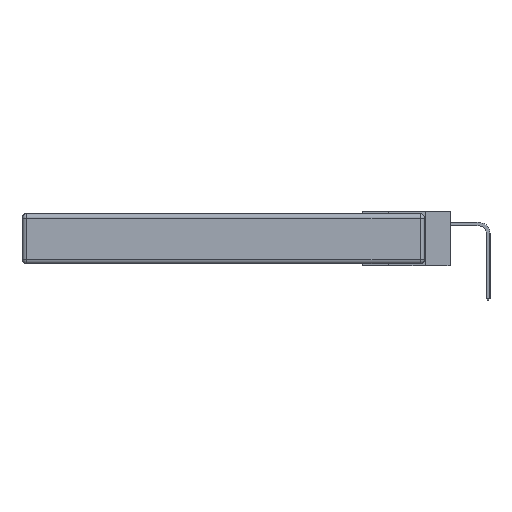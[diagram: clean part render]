
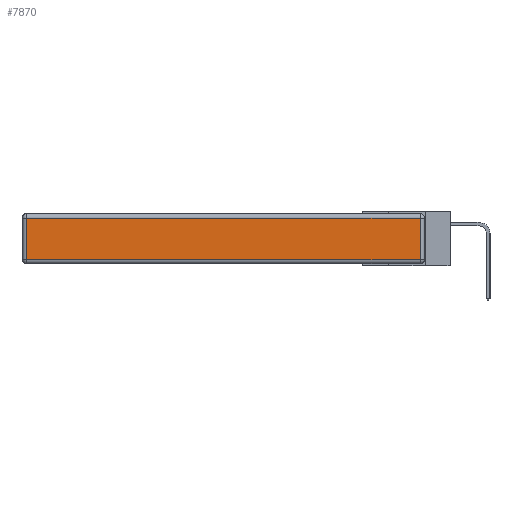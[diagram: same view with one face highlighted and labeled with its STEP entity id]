
A CAD part, left-side view. The second image highlights one B-rep face of the part: STEP entity #7870.
In plain terms, the highlighted planar face has unit normal (-1, 0, 0).
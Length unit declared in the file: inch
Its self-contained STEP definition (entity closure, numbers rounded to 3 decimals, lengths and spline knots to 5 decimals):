
#956 = VECTOR ( 'NONE', #12229, 39.37008 ) ;
#3264 = AXIS2_PLACEMENT_3D ( 'NONE', #3425, #10916, #8335 ) ;
#3312 = PLANE ( 'NONE',  #3264 ) ;
#3425 = CARTESIAN_POINT ( 'NONE',  ( 0., 0., -0.343 ) ) ;
#4411 = CARTESIAN_POINT ( 'NONE',  ( 0., 2.72, -0.03 ) ) ;
#5240 = DIRECTION ( 'NONE',  ( 0., 0., -1. ) ) ;
#5314 = LINE ( 'NONE', #24860, #31729 ) ;
#6458 = ORIENTED_EDGE ( 'NONE', *, *, #26050, .T. ) ;
#7370 = CARTESIAN_POINT ( 'NONE',  ( 0., 2.75, -0.03 ) ) ;
#7870 = ADVANCED_FACE ( 'NONE', ( #29804 ), #3312, .T. ) ;
#8335 = DIRECTION ( 'NONE',  ( 0., 0., 1. ) ) ;
#8623 = LINE ( 'NONE', #7370, #16693 ) ;
#8776 = VERTEX_POINT ( 'NONE', #24275 ) ;
#10916 = DIRECTION ( 'NONE',  ( -1., 0., 0. ) ) ;
#11237 = LINE ( 'NONE', #15755, #22353 ) ;
#12127 = CARTESIAN_POINT ( 'NONE',  ( 0., 0., -0.313 ) ) ;
#12229 = DIRECTION ( 'NONE',  ( 0., -1., 0. ) ) ;
#12957 = VERTEX_POINT ( 'NONE', #16671 ) ;
#13455 = VERTEX_POINT ( 'NONE', #13497 ) ;
#13497 = CARTESIAN_POINT ( 'NONE',  ( 0., 0.03, -0.313 ) ) ;
#15755 = CARTESIAN_POINT ( 'NONE',  ( 0., 0.03, -0.343 ) ) ;
#16356 = VERTEX_POINT ( 'NONE', #4411 ) ;
#16671 = CARTESIAN_POINT ( 'NONE',  ( 0., 0.03, -0.03 ) ) ;
#16693 = VECTOR ( 'NONE', #22162, 39.37008 ) ;
#20023 = ORIENTED_EDGE ( 'NONE', *, *, #26018, .T. ) ;
#20680 = DIRECTION ( 'NONE',  ( 0., 0., 1. ) ) ;
#21507 = ORIENTED_EDGE ( 'NONE', *, *, #23177, .T. ) ;
#22162 = DIRECTION ( 'NONE',  ( 0., 1., 0. ) ) ;
#22353 = VECTOR ( 'NONE', #20680, 39.37008 ) ;
#23177 = EDGE_CURVE ( 'NONE', #16356, #8776, #5314, .T. ) ;
#24275 = CARTESIAN_POINT ( 'NONE',  ( 0., 2.72, -0.313 ) ) ;
#24860 = CARTESIAN_POINT ( 'NONE',  ( 0., 2.72, -0.343 ) ) ;
#25427 = EDGE_LOOP ( 'NONE', ( #20023, #31093, #6458, #21507 ) ) ;
#25518 = LINE ( 'NONE', #12127, #956 ) ;
#26018 = EDGE_CURVE ( 'NONE', #8776, #13455, #25518, .T. ) ;
#26050 = EDGE_CURVE ( 'NONE', #12957, #16356, #8623, .T. ) ;
#27033 = EDGE_CURVE ( 'NONE', #13455, #12957, #11237, .T. ) ;
#29804 = FACE_OUTER_BOUND ( 'NONE', #25427, .T. ) ;
#31093 = ORIENTED_EDGE ( 'NONE', *, *, #27033, .T. ) ;
#31729 = VECTOR ( 'NONE', #5240, 39.37008 ) ;
